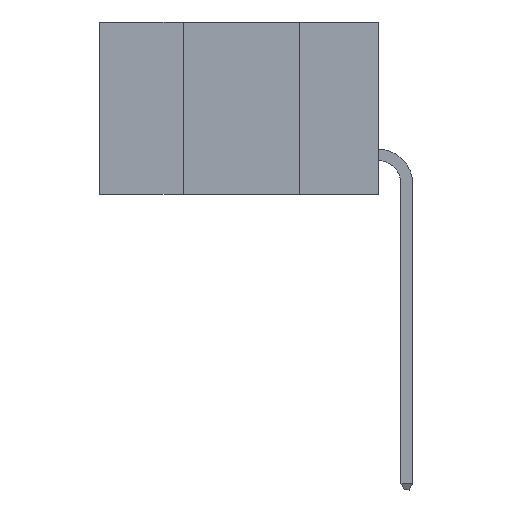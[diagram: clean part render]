
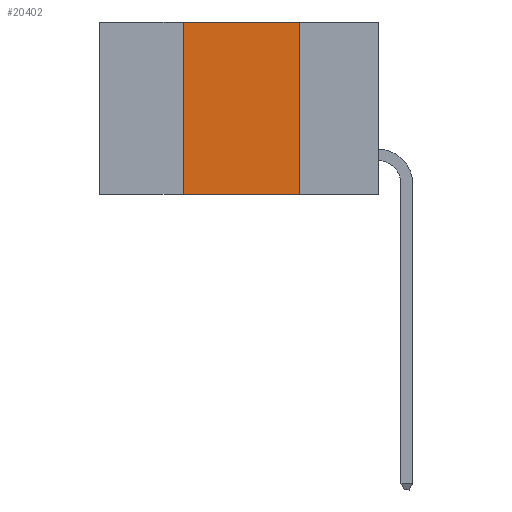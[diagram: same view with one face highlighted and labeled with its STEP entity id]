
A CAD part, left-side view. The second image highlights one B-rep face of the part: STEP entity #20402.
In plain terms, the highlighted planar face has unit normal (-1, 0, 0).
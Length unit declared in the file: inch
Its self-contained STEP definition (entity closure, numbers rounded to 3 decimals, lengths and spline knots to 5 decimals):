
#1171 = DIRECTION ( 'NONE',  ( 0., 0., 1. ) ) ;
#1295 = CARTESIAN_POINT ( 'NONE',  ( 0., 0.42, 0. ) ) ;
#3103 = CARTESIAN_POINT ( 'NONE',  ( 0., 0.42, -0.37 ) ) ;
#3495 = LINE ( 'NONE', #8584, #8060 ) ;
#3633 = LINE ( 'NONE', #22404, #12762 ) ;
#6248 = EDGE_LOOP ( 'NONE', ( #13584, #17123, #14514, #25094 ) ) ;
#6449 = VERTEX_POINT ( 'NONE', #18791 ) ;
#6609 = VECTOR ( 'NONE', #17322, 39.37008 ) ;
#8009 = EDGE_CURVE ( 'NONE', #18616, #8533, #3633, .T. ) ;
#8060 = VECTOR ( 'NONE', #20233, 39.37008 ) ;
#8533 = VERTEX_POINT ( 'NONE', #1295 ) ;
#8584 = CARTESIAN_POINT ( 'NONE',  ( 0., 0.17, 0. ) ) ;
#9491 = DIRECTION ( 'NONE',  ( 0., -1., 0. ) ) ;
#9704 = EDGE_CURVE ( 'NONE', #18616, #6449, #18253, .T. ) ;
#11495 = DIRECTION ( 'NONE',  ( 1., 0., 0. ) ) ;
#12762 = VECTOR ( 'NONE', #1171, 39.37008 ) ;
#13584 = ORIENTED_EDGE ( 'NONE', *, *, #14415, .F. ) ;
#14160 = FACE_OUTER_BOUND ( 'NONE', #6248, .T. ) ;
#14415 = EDGE_CURVE ( 'NONE', #24265, #6449, #3495, .T. ) ;
#14514 = ORIENTED_EDGE ( 'NONE', *, *, #8009, .F. ) ;
#15443 = CARTESIAN_POINT ( 'NONE',  ( 0., 0.6, 0. ) ) ;
#17123 = ORIENTED_EDGE ( 'NONE', *, *, #19247, .F. ) ;
#17322 = DIRECTION ( 'NONE',  ( 0., -1., 0. ) ) ;
#17516 = PLANE ( 'NONE',  #18453 ) ;
#18253 = LINE ( 'NONE', #23082, #6609 ) ;
#18453 = AXIS2_PLACEMENT_3D ( 'NONE', #15443, #11495, #21322 ) ;
#18616 = VERTEX_POINT ( 'NONE', #3103 ) ;
#18791 = CARTESIAN_POINT ( 'NONE',  ( 0., 0.17, -0.37 ) ) ;
#19247 = EDGE_CURVE ( 'NONE', #8533, #24265, #21532, .T. ) ;
#20233 = DIRECTION ( 'NONE',  ( 0., 0., -1. ) ) ;
#20402 = ADVANCED_FACE ( 'NONE', ( #14160 ), #17516, .F. ) ;
#21131 = CARTESIAN_POINT ( 'NONE',  ( 0., 0.6, 0. ) ) ;
#21322 = DIRECTION ( 'NONE',  ( 0., 0., -1. ) ) ;
#21532 = LINE ( 'NONE', #21131, #24898 ) ;
#21822 = CARTESIAN_POINT ( 'NONE',  ( 0., 0.17, 0. ) ) ;
#22404 = CARTESIAN_POINT ( 'NONE',  ( 0., 0.42, 0. ) ) ;
#23082 = CARTESIAN_POINT ( 'NONE',  ( 0., 0.6, -0.37 ) ) ;
#24265 = VERTEX_POINT ( 'NONE', #21822 ) ;
#24898 = VECTOR ( 'NONE', #9491, 39.37008 ) ;
#25094 = ORIENTED_EDGE ( 'NONE', *, *, #9704, .T. ) ;
